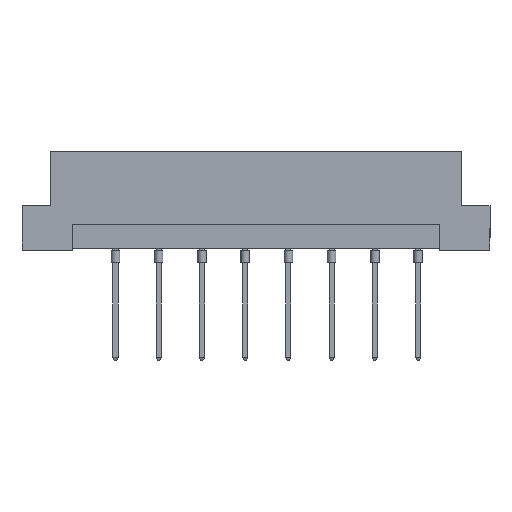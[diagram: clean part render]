
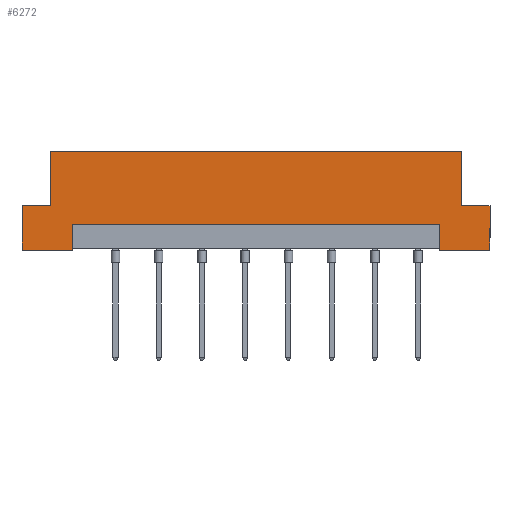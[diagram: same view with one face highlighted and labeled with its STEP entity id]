
A CAD part, front view. The second image highlights one B-rep face of the part: STEP entity #6272.
In plain terms, the highlighted planar face has unit normal (0, -1, 0).
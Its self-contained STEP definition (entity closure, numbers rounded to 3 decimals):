
#52 = LINE ( 'NONE', #4204, #4432 ) ;
#215 = LINE ( 'NONE', #6147, #4108 ) ;
#246 = ORIENTED_EDGE ( 'NONE', *, *, #2448, .T. ) ;
#294 = LINE ( 'NONE', #6320, #3772 ) ;
#419 = LINE ( 'NONE', #1396, #2682 ) ;
#425 = EDGE_CURVE ( 'NONE', #5974, #1104, #6676, .T. ) ;
#464 = CARTESIAN_POINT ( 'NONE',  ( -21.6, -4.3, 3. ) ) ;
#540 = DIRECTION ( 'NONE',  ( 0., 1., 0. ) ) ;
#597 = ORIENTED_EDGE ( 'NONE', *, *, #856, .F. ) ;
#598 = EDGE_CURVE ( 'NONE', #1154, #6853, #419, .T. ) ;
#730 = DIRECTION ( 'NONE',  ( 1., 0., 0. ) ) ;
#740 = ORIENTED_EDGE ( 'NONE', *, *, #3543, .T. ) ;
#789 = CARTESIAN_POINT ( 'NONE',  ( 27.5, -4.3, 5.2 ) ) ;
#856 = EDGE_CURVE ( 'NONE', #1001, #4345, #2483, .T. ) ;
#1001 = VERTEX_POINT ( 'NONE', #2121 ) ;
#1103 = ORIENTED_EDGE ( 'NONE', *, *, #3130, .T. ) ;
#1104 = VERTEX_POINT ( 'NONE', #1657 ) ;
#1154 = VERTEX_POINT ( 'NONE', #4389 ) ;
#1253 = LINE ( 'NONE', #5482, #4655 ) ;
#1396 = CARTESIAN_POINT ( 'NONE',  ( 21.6, -4.3, 0.2 ) ) ;
#1412 = VECTOR ( 'NONE', #3059, 1000. ) ;
#1435 = ORIENTED_EDGE ( 'NONE', *, *, #598, .F. ) ;
#1437 = CARTESIAN_POINT ( 'NONE',  ( 24.2, -4.3, 5.2 ) ) ;
#1504 = DIRECTION ( 'NONE',  ( 1., 0., 0. ) ) ;
#1527 = VECTOR ( 'NONE', #730, 1000. ) ;
#1583 = LINE ( 'NONE', #4765, #3152 ) ;
#1629 = CARTESIAN_POINT ( 'NONE',  ( -21.6, -4.3, 0. ) ) ;
#1657 = CARTESIAN_POINT ( 'NONE',  ( 27.5, -4.3, 0. ) ) ;
#1870 = DIRECTION ( 'NONE',  ( 0., 0., 1. ) ) ;
#1877 = CARTESIAN_POINT ( 'NONE',  ( 21.6, -4.3, 3. ) ) ;
#1878 = ORIENTED_EDGE ( 'NONE', *, *, #3699, .F. ) ;
#2012 = VECTOR ( 'NONE', #6357, 1000. ) ;
#2040 = ORIENTED_EDGE ( 'NONE', *, *, #3456, .T. ) ;
#2051 = CARTESIAN_POINT ( 'NONE',  ( -27.5, -4.3, 5.2 ) ) ;
#2121 = CARTESIAN_POINT ( 'NONE',  ( -24.2, -4.3, 5.2 ) ) ;
#2346 = CARTESIAN_POINT ( 'NONE',  ( 24.2, -4.3, 11.6 ) ) ;
#2391 = CARTESIAN_POINT ( 'NONE',  ( 27.5, -4.3, 11.6 ) ) ;
#2448 = EDGE_CURVE ( 'NONE', #1154, #1104, #4788, .T. ) ;
#2483 = LINE ( 'NONE', #6166, #5020 ) ;
#2682 = VECTOR ( 'NONE', #4692, 1000. ) ;
#2756 = PLANE ( 'NONE',  #6673 ) ;
#2765 = CARTESIAN_POINT ( 'NONE',  ( 27.5, -4.3, 0. ) ) ;
#2844 = LINE ( 'NONE', #4477, #1527 ) ;
#2879 = DIRECTION ( 'NONE',  ( 0., 0., -1. ) ) ;
#3008 = VECTOR ( 'NONE', #2879, 1000. ) ;
#3059 = DIRECTION ( 'NONE',  ( 0., 0., -1. ) ) ;
#3130 = EDGE_CURVE ( 'NONE', #3522, #6884, #1583, .T. ) ;
#3152 = VECTOR ( 'NONE', #4203, 1000. ) ;
#3281 = VERTEX_POINT ( 'NONE', #4410 ) ;
#3456 = EDGE_CURVE ( 'NONE', #3281, #6853, #4167, .T. ) ;
#3499 = CARTESIAN_POINT ( 'NONE',  ( -24.2, -4.3, 11.6 ) ) ;
#3522 = VERTEX_POINT ( 'NONE', #1437 ) ;
#3543 = EDGE_CURVE ( 'NONE', #4353, #5548, #3579, .T. ) ;
#3579 = LINE ( 'NONE', #4093, #1412 ) ;
#3658 = EDGE_LOOP ( 'NONE', ( #2040, #1435, #246, #4128, #4838, #1103, #5367, #597, #1878, #740, #6655, #6511 ) ) ;
#3699 = EDGE_CURVE ( 'NONE', #4353, #1001, #2844, .T. ) ;
#3750 = DIRECTION ( 'NONE',  ( -1., 0., 0. ) ) ;
#3772 = VECTOR ( 'NONE', #4228, 1000. ) ;
#3904 = CARTESIAN_POINT ( 'NONE',  ( -27.5, -4.3, 0. ) ) ;
#4093 = CARTESIAN_POINT ( 'NONE',  ( -27.5, -4.3, 11.6 ) ) ;
#4108 = VECTOR ( 'NONE', #4436, 1000. ) ;
#4128 = ORIENTED_EDGE ( 'NONE', *, *, #425, .F. ) ;
#4167 = LINE ( 'NONE', #464, #4433 ) ;
#4203 = DIRECTION ( 'NONE',  ( 0., 0., 1. ) ) ;
#4204 = CARTESIAN_POINT ( 'NONE',  ( 27.5, -4.3, 0. ) ) ;
#4228 = DIRECTION ( 'NONE',  ( 1., 0., 0. ) ) ;
#4311 = DIRECTION ( 'NONE',  ( 1., 0., 0. ) ) ;
#4345 = VERTEX_POINT ( 'NONE', #3499 ) ;
#4353 = VERTEX_POINT ( 'NONE', #2051 ) ;
#4389 = CARTESIAN_POINT ( 'NONE',  ( 21.6, -4.3, 0. ) ) ;
#4410 = CARTESIAN_POINT ( 'NONE',  ( -21.6, -4.3, 3. ) ) ;
#4432 = VECTOR ( 'NONE', #4311, 1000. ) ;
#4433 = VECTOR ( 'NONE', #1504, 1000. ) ;
#4436 = DIRECTION ( 'NONE',  ( 1., 0., 0. ) ) ;
#4477 = CARTESIAN_POINT ( 'NONE',  ( -27.5, -4.3, 5.2 ) ) ;
#4655 = VECTOR ( 'NONE', #6066, 1000. ) ;
#4692 = DIRECTION ( 'NONE',  ( 0., 0., 1. ) ) ;
#4765 = CARTESIAN_POINT ( 'NONE',  ( 24.2, -4.3, 5.2 ) ) ;
#4788 = LINE ( 'NONE', #2765, #2012 ) ;
#4838 = ORIENTED_EDGE ( 'NONE', *, *, #6499, .F. ) ;
#4873 = CARTESIAN_POINT ( 'NONE',  ( 27.5, -4.3, 11.6 ) ) ;
#5020 = VECTOR ( 'NONE', #1870, 1000. ) ;
#5037 = EDGE_CURVE ( 'NONE', #4345, #6884, #215, .T. ) ;
#5324 = FACE_OUTER_BOUND ( 'NONE', #3658, .T. ) ;
#5367 = ORIENTED_EDGE ( 'NONE', *, *, #5037, .F. ) ;
#5448 = EDGE_CURVE ( 'NONE', #3281, #6666, #1253, .T. ) ;
#5482 = CARTESIAN_POINT ( 'NONE',  ( -21.6, -4.3, 0.2 ) ) ;
#5548 = VERTEX_POINT ( 'NONE', #3904 ) ;
#5974 = VERTEX_POINT ( 'NONE', #789 ) ;
#6066 = DIRECTION ( 'NONE',  ( 0., 0., -1. ) ) ;
#6147 = CARTESIAN_POINT ( 'NONE',  ( 27.5, -4.3, 11.6 ) ) ;
#6166 = CARTESIAN_POINT ( 'NONE',  ( -24.2, -4.3, 5.2 ) ) ;
#6176 = EDGE_CURVE ( 'NONE', #5548, #6666, #52, .T. ) ;
#6272 = ADVANCED_FACE ( 'NONE', ( #5324 ), #2756, .F. ) ;
#6320 = CARTESIAN_POINT ( 'NONE',  ( 27.5, -4.3, 5.2 ) ) ;
#6357 = DIRECTION ( 'NONE',  ( 1., 0., 0. ) ) ;
#6499 = EDGE_CURVE ( 'NONE', #3522, #5974, #294, .T. ) ;
#6511 = ORIENTED_EDGE ( 'NONE', *, *, #5448, .F. ) ;
#6655 = ORIENTED_EDGE ( 'NONE', *, *, #6176, .T. ) ;
#6666 = VERTEX_POINT ( 'NONE', #1629 ) ;
#6673 = AXIS2_PLACEMENT_3D ( 'NONE', #4873, #540, #3750 ) ;
#6676 = LINE ( 'NONE', #2391, #3008 ) ;
#6853 = VERTEX_POINT ( 'NONE', #1877 ) ;
#6884 = VERTEX_POINT ( 'NONE', #2346 ) ;
